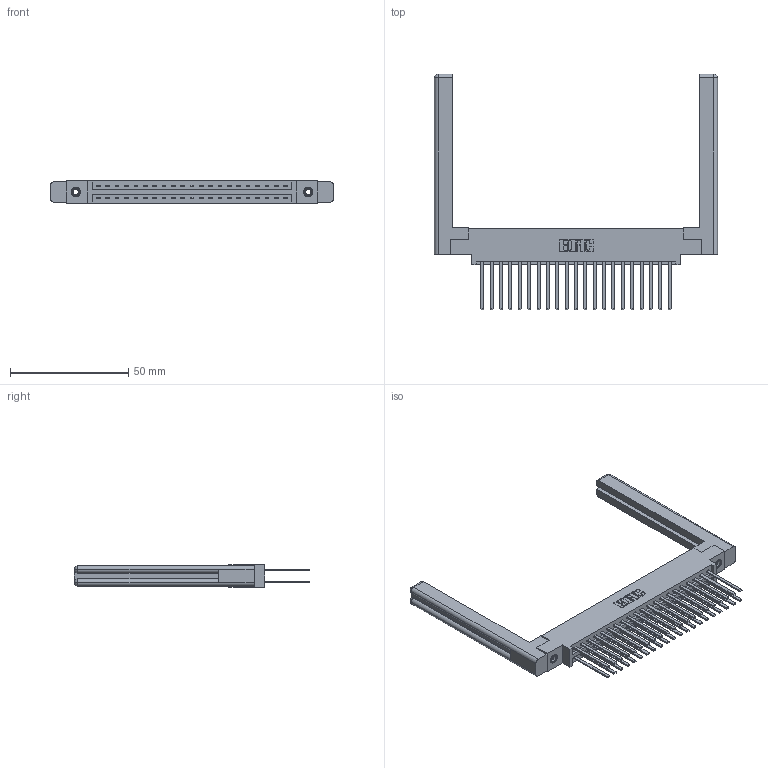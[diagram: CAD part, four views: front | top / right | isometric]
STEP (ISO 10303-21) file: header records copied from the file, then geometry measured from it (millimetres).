
FILE_DESCRIPTION (( 'STEP AP203' ), '1' );
FILE_NAME ('337-042-544-858.STEP', '2019-10-11T12:59:03', ( '' ), ( '' ), 'SwSTEP 2.0', 'SolidWorks 2016', '' );
FILE_SCHEMA (( 'CONFIG_CONTROL_DESIGN' ));
Length unit declared in the file: inch
Products named in the file (5): 337 Part_0.170 Offset - 0.156 Dia-TI; 345-292-001_345-293-144; 345-250-001_345-250-001-102; 337-042-544-858; 307-220-058
Assembly tree (47 placements, depth 2):
  337-042-544-858
    337 Part_0.170 Offset - 0.156 Dia-TI
    345-292-001_345-293-144  x42
    345-250-001_345-250-001-102  x2
    307-220-058  x2
Bounding box: 119.84 x 99.7 x 9.4 mm (x, y, z)
Volume: 19963.5 mm3; surface area: 21368.2 mm2
Topology: 47 solids, 47 shells, 2276 faces, 6683 edges, 4386 vertices
Faces by surface type: plane 1586, cylinder 666, cone 12, torus 12
Entity records: 21580 total; most frequent: CARTESIAN_POINT 3661, ORIENTED_EDGE 3536, DIRECTION 3164, EDGE_CURVE 1768, VECTOR 1596, LINE 1596, VERTEX_POINT 1170, AXIS2_PLACEMENT_3D 784
